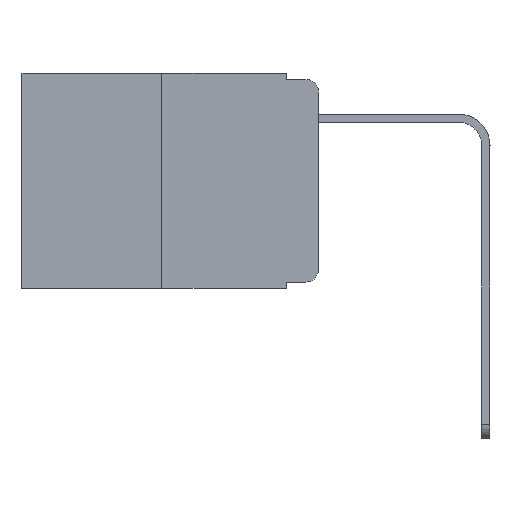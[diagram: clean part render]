
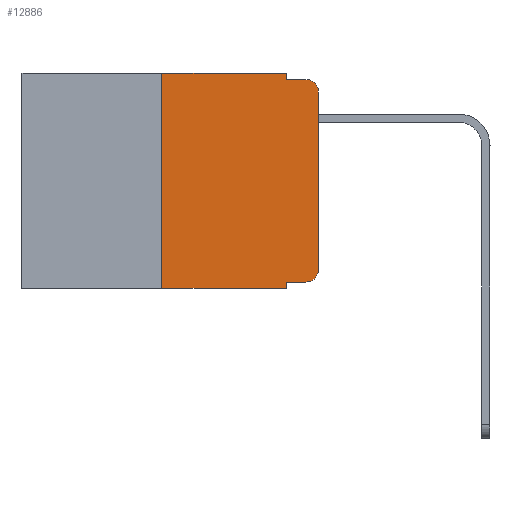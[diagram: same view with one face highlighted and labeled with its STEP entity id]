
A CAD part, left-side view. The second image highlights one B-rep face of the part: STEP entity #12886.
In plain terms, the highlighted planar face has unit normal (-1, 0, 0).
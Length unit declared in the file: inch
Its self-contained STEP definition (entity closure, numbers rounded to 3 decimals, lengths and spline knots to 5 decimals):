
#123 = ORIENTED_EDGE ( 'NONE', *, *, #4790, .F. ) ;
#603 = DIRECTION ( 'NONE',  ( 0., -1., 0. ) ) ;
#772 = CARTESIAN_POINT ( 'NONE',  ( 0., 0.25, -0.343 ) ) ;
#1146 = VERTEX_POINT ( 'NONE', #11020 ) ;
#1918 = CARTESIAN_POINT ( 'NONE',  ( 0., 0.25, 0. ) ) ;
#1942 = LINE ( 'NONE', #10383, #13358 ) ;
#2043 = DIRECTION ( 'NONE',  ( -1., 0., 0. ) ) ;
#2086 = CARTESIAN_POINT ( 'NONE',  ( 0., 0.02, -0.313 ) ) ;
#2103 = VECTOR ( 'NONE', #5503, 39.37008 ) ;
#2283 = ORIENTED_EDGE ( 'NONE', *, *, #14693, .T. ) ;
#3328 = CARTESIAN_POINT ( 'NONE',  ( 0., 0.051, -0.01 ) ) ;
#3436 = VERTEX_POINT ( 'NONE', #15514 ) ;
#3627 = AXIS2_PLACEMENT_3D ( 'NONE', #15719, #2043, #4921 ) ;
#3687 = CARTESIAN_POINT ( 'NONE',  ( 0., 0.25, 0. ) ) ;
#3688 = DIRECTION ( 'NONE',  ( -1., 0., 0. ) ) ;
#4224 = LINE ( 'NONE', #1918, #12774 ) ;
#4677 = EDGE_CURVE ( 'NONE', #9735, #17537, #5898, .T. ) ;
#4714 = DIRECTION ( 'NONE',  ( 0., 0., -1. ) ) ;
#4767 = ORIENTED_EDGE ( 'NONE', *, *, #17371, .T. ) ;
#4790 = EDGE_CURVE ( 'NONE', #11152, #10396, #7971, .T. ) ;
#4921 = DIRECTION ( 'NONE',  ( 0., 0., -1. ) ) ;
#5358 = LINE ( 'NONE', #15339, #7929 ) ;
#5413 = AXIS2_PLACEMENT_3D ( 'NONE', #19274, #5718, #7161 ) ;
#5457 = ORIENTED_EDGE ( 'NONE', *, *, #4677, .F. ) ;
#5474 = CARTESIAN_POINT ( 'NONE',  ( 0., 0.02, -0.01 ) ) ;
#5503 = DIRECTION ( 'NONE',  ( 0., 0., 1. ) ) ;
#5718 = DIRECTION ( 'NONE',  ( 1., 0., 0. ) ) ;
#5742 = VERTEX_POINT ( 'NONE', #3687 ) ;
#5898 = LINE ( 'NONE', #3328, #12089 ) ;
#6040 = FACE_OUTER_BOUND ( 'NONE', #10785, .T. ) ;
#6071 = VERTEX_POINT ( 'NONE', #13945 ) ;
#6355 = CARTESIAN_POINT ( 'NONE',  ( 0., 0.051, 0. ) ) ;
#6549 = DIRECTION ( 'NONE',  ( 0., 0., -1. ) ) ;
#7135 = CARTESIAN_POINT ( 'NONE',  ( 0., 0., 0. ) ) ;
#7161 = DIRECTION ( 'NONE',  ( 0., 0., -1. ) ) ;
#7929 = VECTOR ( 'NONE', #13882, 39.37008 ) ;
#7971 = LINE ( 'NONE', #19204, #7990 ) ;
#7990 = VECTOR ( 'NONE', #11570, 39.37008 ) ;
#8318 = VECTOR ( 'NONE', #4714, 39.37008 ) ;
#8419 = CARTESIAN_POINT ( 'NONE',  ( 0., 0.473, -0.343 ) ) ;
#8503 = ORIENTED_EDGE ( 'NONE', *, *, #9681, .F. ) ;
#8660 = EDGE_CURVE ( 'NONE', #1146, #19622, #11641, .T. ) ;
#8758 = DIRECTION ( 'NONE',  ( 0., -1., 0. ) ) ;
#9681 = EDGE_CURVE ( 'NONE', #14115, #5742, #4224, .T. ) ;
#9735 = VERTEX_POINT ( 'NONE', #11241 ) ;
#10172 = PLANE ( 'NONE',  #5413 ) ;
#10383 = CARTESIAN_POINT ( 'NONE',  ( 0., 0.473, 0. ) ) ;
#10396 = VERTEX_POINT ( 'NONE', #11425 ) ;
#10785 = EDGE_LOOP ( 'NONE', ( #13327, #18473, #5457, #17611, #13803, #8503, #4767, #123, #11754, #2283 ) ) ;
#11003 = LINE ( 'NONE', #8419, #16450 ) ;
#11013 = EDGE_CURVE ( 'NONE', #5742, #3436, #1942, .T. ) ;
#11020 = CARTESIAN_POINT ( 'NONE',  ( 0., 0., -0.313 ) ) ;
#11152 = VERTEX_POINT ( 'NONE', #18104 ) ;
#11241 = CARTESIAN_POINT ( 'NONE',  ( 0., 0.051, -0.01 ) ) ;
#11425 = CARTESIAN_POINT ( 'NONE',  ( 0., 0.051, -0.343 ) ) ;
#11570 = DIRECTION ( 'NONE',  ( 0., 0., -1. ) ) ;
#11641 = LINE ( 'NONE', #7135, #2103 ) ;
#11754 = ORIENTED_EDGE ( 'NONE', *, *, #12436, .T. ) ;
#11933 = AXIS2_PLACEMENT_3D ( 'NONE', #2086, #3688, #6549 ) ;
#12089 = VECTOR ( 'NONE', #15865, 39.37008 ) ;
#12436 = EDGE_CURVE ( 'NONE', #11152, #6071, #5358, .T. ) ;
#12774 = VECTOR ( 'NONE', #17176, 39.37008 ) ;
#12886 = ADVANCED_FACE ( 'NONE', ( #6040 ), #10172, .F. ) ;
#13139 = EDGE_CURVE ( 'NONE', #19622, #17537, #17400, .T. ) ;
#13327 = ORIENTED_EDGE ( 'NONE', *, *, #8660, .T. ) ;
#13358 = VECTOR ( 'NONE', #8758, 39.37008 ) ;
#13803 = ORIENTED_EDGE ( 'NONE', *, *, #11013, .F. ) ;
#13882 = DIRECTION ( 'NONE',  ( 0., -1., 0. ) ) ;
#13945 = CARTESIAN_POINT ( 'NONE',  ( 0., 0.02, -0.333 ) ) ;
#14115 = VERTEX_POINT ( 'NONE', #772 ) ;
#14693 = EDGE_CURVE ( 'NONE', #6071, #1146, #18290, .T. ) ;
#14961 = CARTESIAN_POINT ( 'NONE',  ( 0., 0., -0.03 ) ) ;
#15339 = CARTESIAN_POINT ( 'NONE',  ( 0., 0.051, -0.333 ) ) ;
#15452 = LINE ( 'NONE', #6355, #8318 ) ;
#15514 = CARTESIAN_POINT ( 'NONE',  ( 0., 0.051, 0. ) ) ;
#15719 = CARTESIAN_POINT ( 'NONE',  ( 0., 0.02, -0.03 ) ) ;
#15865 = DIRECTION ( 'NONE',  ( 0., -1., 0. ) ) ;
#16450 = VECTOR ( 'NONE', #603, 39.37008 ) ;
#17176 = DIRECTION ( 'NONE',  ( 0., 0., 1. ) ) ;
#17371 = EDGE_CURVE ( 'NONE', #14115, #10396, #11003, .T. ) ;
#17400 = CIRCLE ( 'NONE', #3627, 0.02 ) ;
#17537 = VERTEX_POINT ( 'NONE', #5474 ) ;
#17611 = ORIENTED_EDGE ( 'NONE', *, *, #18267, .F. ) ;
#18104 = CARTESIAN_POINT ( 'NONE',  ( 0., 0.051, -0.333 ) ) ;
#18267 = EDGE_CURVE ( 'NONE', #3436, #9735, #15452, .T. ) ;
#18290 = CIRCLE ( 'NONE', #11933, 0.02 ) ;
#18473 = ORIENTED_EDGE ( 'NONE', *, *, #13139, .T. ) ;
#19204 = CARTESIAN_POINT ( 'NONE',  ( 0., 0.051, 0. ) ) ;
#19274 = CARTESIAN_POINT ( 'NONE',  ( 0., 0.473, 0. ) ) ;
#19622 = VERTEX_POINT ( 'NONE', #14961 ) ;
